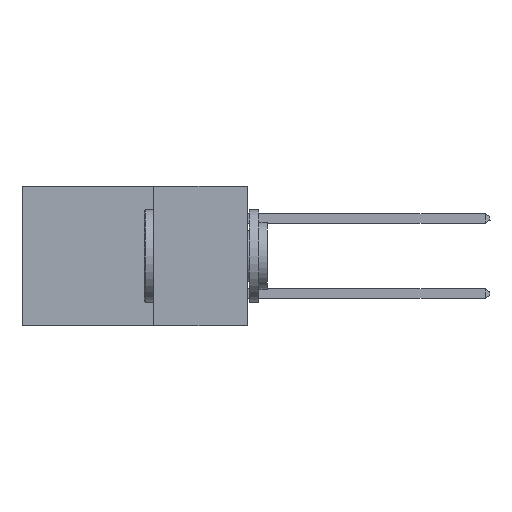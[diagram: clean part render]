
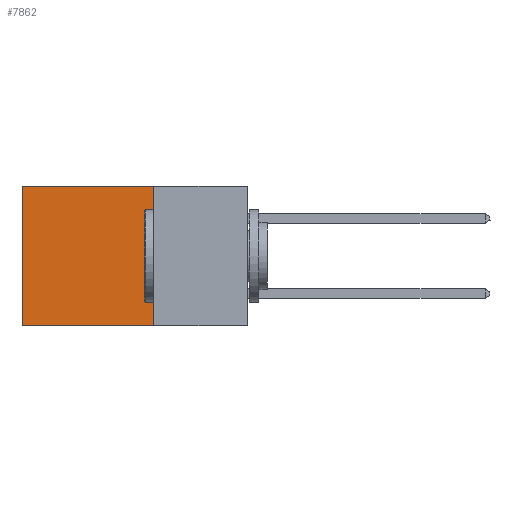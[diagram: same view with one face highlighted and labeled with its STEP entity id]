
A CAD part, left-side view. The second image highlights one B-rep face of the part: STEP entity #7862.
In plain terms, the highlighted planar face has unit normal (-1, 0, 0).
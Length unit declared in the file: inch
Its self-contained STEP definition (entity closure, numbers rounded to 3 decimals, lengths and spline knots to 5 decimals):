
#941 = CARTESIAN_POINT ( 'NONE',  ( 0.2615, 0.6, -0.37 ) ) ;
#1513 = ORIENTED_EDGE ( 'NONE', *, *, #8667, .T. ) ;
#2772 = DIRECTION ( 'NONE',  ( 0., 0., -1. ) ) ;
#3039 = CARTESIAN_POINT ( 'NONE',  ( 0.2615, 0.25, -0.37 ) ) ;
#3452 = VECTOR ( 'NONE', #10585, 39.37008 ) ;
#4331 = ORIENTED_EDGE ( 'NONE', *, *, #17273, .F. ) ;
#4610 = VECTOR ( 'NONE', #6564, 39.37008 ) ;
#4971 = ORIENTED_EDGE ( 'NONE', *, *, #9414, .F. ) ;
#6385 = VERTEX_POINT ( 'NONE', #19374 ) ;
#6564 = DIRECTION ( 'NONE',  ( 0., 1., 0. ) ) ;
#6797 = FACE_OUTER_BOUND ( 'NONE', #7190, .T. ) ;
#7190 = EDGE_LOOP ( 'NONE', ( #1513, #4331, #4971, #8472 ) ) ;
#7309 = LINE ( 'NONE', #3039, #11533 ) ;
#7862 = ADVANCED_FACE ( 'NONE', ( #6797 ), #12660, .F. ) ;
#8472 = ORIENTED_EDGE ( 'NONE', *, *, #12087, .T. ) ;
#8667 = EDGE_CURVE ( 'NONE', #17084, #9743, #8771, .T. ) ;
#8771 = LINE ( 'NONE', #941, #17661 ) ;
#9414 = EDGE_CURVE ( 'NONE', #6385, #11341, #7309, .T. ) ;
#9743 = VERTEX_POINT ( 'NONE', #14650 ) ;
#10034 = LINE ( 'NONE', #11908, #4610 ) ;
#10138 = CARTESIAN_POINT ( 'NONE',  ( 0.2615, 0.25, -0.37 ) ) ;
#10585 = DIRECTION ( 'NONE',  ( 0., 1., 0. ) ) ;
#11341 = VERTEX_POINT ( 'NONE', #10138 ) ;
#11533 = VECTOR ( 'NONE', #17412, 39.37008 ) ;
#11908 = CARTESIAN_POINT ( 'NONE',  ( 0.2615, 0.25, -0.37 ) ) ;
#12034 = DIRECTION ( 'NONE',  ( 0., 0., -1. ) ) ;
#12087 = EDGE_CURVE ( 'NONE', #6385, #17084, #22378, .T. ) ;
#12145 = CARTESIAN_POINT ( 'NONE',  ( 0.2615, 0.25, -0.37 ) ) ;
#12174 = DIRECTION ( 'NONE',  ( 1., 0., 0. ) ) ;
#12660 = PLANE ( 'NONE',  #13160 ) ;
#13160 = AXIS2_PLACEMENT_3D ( 'NONE', #12145, #12174, #12034 ) ;
#14650 = CARTESIAN_POINT ( 'NONE',  ( 0.2615, 0.6, -0.37 ) ) ;
#15041 = CARTESIAN_POINT ( 'NONE',  ( 0.2615, 0.6, 0. ) ) ;
#17084 = VERTEX_POINT ( 'NONE', #15041 ) ;
#17273 = EDGE_CURVE ( 'NONE', #11341, #9743, #10034, .T. ) ;
#17412 = DIRECTION ( 'NONE',  ( 0., 0., -1. ) ) ;
#17661 = VECTOR ( 'NONE', #2772, 39.37008 ) ;
#19374 = CARTESIAN_POINT ( 'NONE',  ( 0.2615, 0.25, 0. ) ) ;
#19406 = CARTESIAN_POINT ( 'NONE',  ( 0.2615, 0.25, 0. ) ) ;
#22378 = LINE ( 'NONE', #19406, #3452 ) ;
